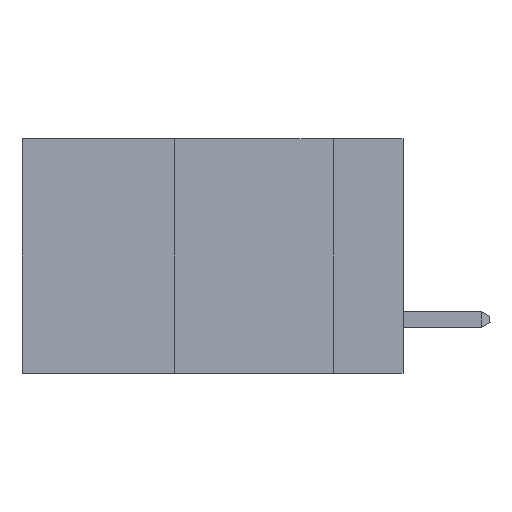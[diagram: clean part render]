
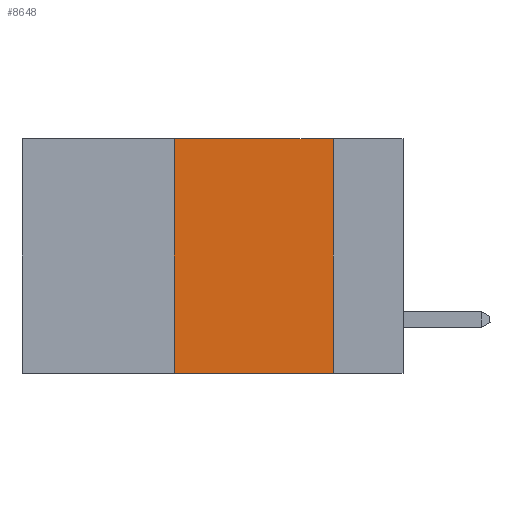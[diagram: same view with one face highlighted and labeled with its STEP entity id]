
A CAD part, left-side view. The second image highlights one B-rep face of the part: STEP entity #8648.
In plain terms, the highlighted planar face has unit normal (-1, 0, 0).
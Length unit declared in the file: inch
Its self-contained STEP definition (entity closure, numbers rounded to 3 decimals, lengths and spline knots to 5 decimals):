
#699 = EDGE_CURVE ( 'NONE', #5726, #18847, #19543, .T. ) ;
#2831 = DIRECTION ( 'NONE',  ( 0., 0., -1. ) ) ;
#3156 = EDGE_CURVE ( 'NONE', #17745, #5726, #21793, .T. ) ;
#4080 = EDGE_CURVE ( 'NONE', #18847, #20054, #17490, .T. ) ;
#4158 = DIRECTION ( 'NONE',  ( 0., -1., 0. ) ) ;
#4511 = CARTESIAN_POINT ( 'NONE',  ( 0., 0.11, 0. ) ) ;
#5287 = PLANE ( 'NONE',  #12983 ) ;
#5317 = FACE_OUTER_BOUND ( 'NONE', #5928, .T. ) ;
#5399 = VECTOR ( 'NONE', #4158, 39.37008 ) ;
#5726 = VERTEX_POINT ( 'NONE', #9561 ) ;
#5928 = EDGE_LOOP ( 'NONE', ( #23379, #10755, #9610, #16429 ) ) ;
#8648 = ADVANCED_FACE ( 'NONE', ( #5317 ), #5287, .F. ) ;
#9561 = CARTESIAN_POINT ( 'NONE',  ( 0., 0.36, 0. ) ) ;
#9610 = ORIENTED_EDGE ( 'NONE', *, *, #3156, .F. ) ;
#9817 = CARTESIAN_POINT ( 'NONE',  ( 0., 0.36, -0.37 ) ) ;
#9885 = CARTESIAN_POINT ( 'NONE',  ( 0., 0.6, -0.37 ) ) ;
#10755 = ORIENTED_EDGE ( 'NONE', *, *, #699, .F. ) ;
#12523 = EDGE_CURVE ( 'NONE', #17745, #20054, #17485, .T. ) ;
#12983 = AXIS2_PLACEMENT_3D ( 'NONE', #20999, #24189, #2831 ) ;
#14546 = VECTOR ( 'NONE', #24637, 39.37008 ) ;
#14821 = CARTESIAN_POINT ( 'NONE',  ( 0., 0.36, 0. ) ) ;
#16429 = ORIENTED_EDGE ( 'NONE', *, *, #12523, .T. ) ;
#16713 = CARTESIAN_POINT ( 'NONE',  ( 0., 0.11, -0.37 ) ) ;
#17485 = LINE ( 'NONE', #9885, #5399 ) ;
#17490 = LINE ( 'NONE', #4511, #21800 ) ;
#17745 = VERTEX_POINT ( 'NONE', #9817 ) ;
#18847 = VERTEX_POINT ( 'NONE', #24095 ) ;
#19543 = LINE ( 'NONE', #19777, #21343 ) ;
#19777 = CARTESIAN_POINT ( 'NONE',  ( 0., 0.6, 0. ) ) ;
#19946 = DIRECTION ( 'NONE',  ( 0., -1., 0. ) ) ;
#20054 = VERTEX_POINT ( 'NONE', #16713 ) ;
#20999 = CARTESIAN_POINT ( 'NONE',  ( 0., 0.6, 0. ) ) ;
#21343 = VECTOR ( 'NONE', #19946, 39.37008 ) ;
#21793 = LINE ( 'NONE', #14821, #14546 ) ;
#21800 = VECTOR ( 'NONE', #21905, 39.37008 ) ;
#21905 = DIRECTION ( 'NONE',  ( 0., 0., -1. ) ) ;
#23379 = ORIENTED_EDGE ( 'NONE', *, *, #4080, .F. ) ;
#24095 = CARTESIAN_POINT ( 'NONE',  ( 0., 0.11, 0. ) ) ;
#24189 = DIRECTION ( 'NONE',  ( 1., 0., 0. ) ) ;
#24637 = DIRECTION ( 'NONE',  ( 0., 0., 1. ) ) ;
